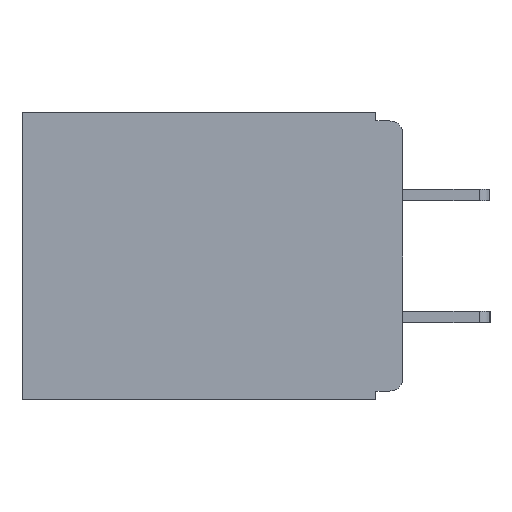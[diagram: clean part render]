
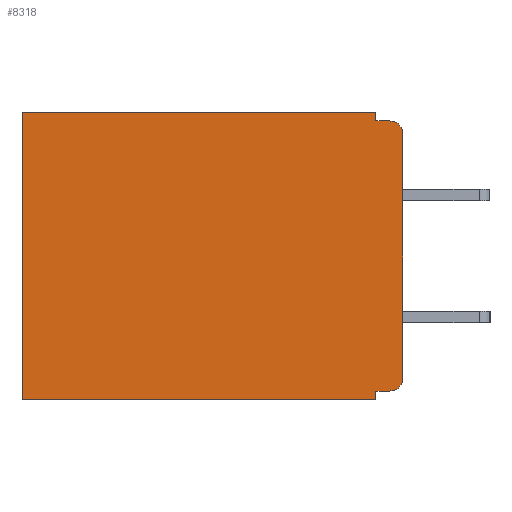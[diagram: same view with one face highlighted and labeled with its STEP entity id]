
A CAD part, left-side view. The second image highlights one B-rep face of the part: STEP entity #8318.
In plain terms, the highlighted planar face has unit normal (-1, 0, 0).
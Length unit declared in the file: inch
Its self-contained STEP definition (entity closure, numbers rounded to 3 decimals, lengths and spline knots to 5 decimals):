
#74 = CARTESIAN_POINT ( 'NONE',  ( 0.3, 0., -0.33 ) ) ;
#298 = ORIENTED_EDGE ( 'NONE', *, *, #14589, .F. ) ;
#323 = FACE_OUTER_BOUND ( 'NONE', #11181, .T. ) ;
#492 = CARTESIAN_POINT ( 'NONE',  ( 0.3, 0., 0. ) ) ;
#523 = DIRECTION ( 'NONE',  ( 0., 1., 0. ) ) ;
#769 = ORIENTED_EDGE ( 'NONE', *, *, #10823, .F. ) ;
#1187 = VERTEX_POINT ( 'NONE', #15953 ) ;
#1248 = ORIENTED_EDGE ( 'NONE', *, *, #4024, .T. ) ;
#2426 = ORIENTED_EDGE ( 'NONE', *, *, #8956, .T. ) ;
#2644 = VERTEX_POINT ( 'NONE', #4671 ) ;
#2681 = VERTEX_POINT ( 'NONE', #17995 ) ;
#2886 = ORIENTED_EDGE ( 'NONE', *, *, #8099, .F. ) ;
#3091 = VECTOR ( 'NONE', #6693, 39.37008 ) ;
#3391 = EDGE_CURVE ( 'NONE', #1187, #2681, #7046, .T. ) ;
#3652 = EDGE_CURVE ( 'NONE', #16773, #4041, #7027, .T. ) ;
#3713 = DIRECTION ( 'NONE',  ( 0., 0., -1. ) ) ;
#3838 = CARTESIAN_POINT ( 'NONE',  ( 0.3, 0.437, -0.33 ) ) ;
#4024 = EDGE_CURVE ( 'NONE', #2644, #4041, #8364, .T. ) ;
#4041 = VERTEX_POINT ( 'NONE', #16017 ) ;
#4089 = VECTOR ( 'NONE', #11317, 39.37008 ) ;
#4608 = VECTOR ( 'NONE', #8667, 39.37008 ) ;
#4671 = CARTESIAN_POINT ( 'NONE',  ( 0.3, 0.015, -0.32 ) ) ;
#5006 = VERTEX_POINT ( 'NONE', #17728 ) ;
#5085 = LINE ( 'NONE', #18104, #4608 ) ;
#5530 = EDGE_CURVE ( 'NONE', #2681, #14170, #16859, .T. ) ;
#5645 = DIRECTION ( 'NONE',  ( 0., 0., -1. ) ) ;
#6138 = DIRECTION ( 'NONE',  ( 0., 1., 0. ) ) ;
#6177 = EDGE_CURVE ( 'NONE', #14792, #16136, #17452, .T. ) ;
#6693 = DIRECTION ( 'NONE',  ( 0., 1., 0. ) ) ;
#7027 = LINE ( 'NONE', #74, #10357 ) ;
#7046 = LINE ( 'NONE', #492, #3091 ) ;
#7137 = CARTESIAN_POINT ( 'NONE',  ( 0.3, 0.031, -0.33 ) ) ;
#7290 = ORIENTED_EDGE ( 'NONE', *, *, #3391, .T. ) ;
#7534 = DIRECTION ( 'NONE',  ( 0., 0., -1. ) ) ;
#7620 = DIRECTION ( 'NONE',  ( 1., 0., 0. ) ) ;
#7642 = LINE ( 'NONE', #17520, #17646 ) ;
#7730 = CARTESIAN_POINT ( 'NONE',  ( 0.3, 0., -0.33 ) ) ;
#7813 = PLANE ( 'NONE',  #13607 ) ;
#8099 = EDGE_CURVE ( 'NONE', #1187, #12750, #11316, .T. ) ;
#8203 = LINE ( 'NONE', #14498, #15107 ) ;
#8318 = ADVANCED_FACE ( 'NONE', ( #323 ), #7813, .F. ) ;
#8364 = CIRCLE ( 'NONE', #11040, 0.015 ) ;
#8667 = DIRECTION ( 'NONE',  ( 0., -1., 0. ) ) ;
#8891 = CIRCLE ( 'NONE', #14738, 0.015 ) ;
#8956 = EDGE_CURVE ( 'NONE', #16773, #5006, #8891, .T. ) ;
#10357 = VECTOR ( 'NONE', #16633, 39.37008 ) ;
#10823 = EDGE_CURVE ( 'NONE', #2644, #14792, #8203, .T. ) ;
#11040 = AXIS2_PLACEMENT_3D ( 'NONE', #18044, #11717, #16079 ) ;
#11181 = EDGE_LOOP ( 'NONE', ( #16941, #2426, #17340, #2886, #7290, #18146, #298, #11937, #769, #1248 ) ) ;
#11316 = LINE ( 'NONE', #11357, #4089 ) ;
#11317 = DIRECTION ( 'NONE',  ( 0., 0., -1. ) ) ;
#11357 = CARTESIAN_POINT ( 'NONE',  ( 0.3, 0.031, 0. ) ) ;
#11717 = DIRECTION ( 'NONE',  ( -1., 0., 0. ) ) ;
#11937 = ORIENTED_EDGE ( 'NONE', *, *, #6177, .F. ) ;
#12648 = CARTESIAN_POINT ( 'NONE',  ( 0.3, 0.437, -0.33 ) ) ;
#12750 = VERTEX_POINT ( 'NONE', #14842 ) ;
#13193 = CARTESIAN_POINT ( 'NONE',  ( 0.3, 0.031, -0.33 ) ) ;
#13607 = AXIS2_PLACEMENT_3D ( 'NONE', #7730, #7620, #7534 ) ;
#13959 = VECTOR ( 'NONE', #5645, 39.37008 ) ;
#14170 = VERTEX_POINT ( 'NONE', #12648 ) ;
#14191 = VECTOR ( 'NONE', #3713, 39.37008 ) ;
#14498 = CARTESIAN_POINT ( 'NONE',  ( 0.3, 0., -0.32 ) ) ;
#14589 = EDGE_CURVE ( 'NONE', #16136, #14170, #7642, .T. ) ;
#14738 = AXIS2_PLACEMENT_3D ( 'NONE', #15737, #15732, #15708 ) ;
#14792 = VERTEX_POINT ( 'NONE', #15356 ) ;
#14842 = CARTESIAN_POINT ( 'NONE',  ( 0.3, 0.031, -0.01 ) ) ;
#15107 = VECTOR ( 'NONE', #6138, 39.37008 ) ;
#15149 = CARTESIAN_POINT ( 'NONE',  ( 0.3, 0., -0.025 ) ) ;
#15356 = CARTESIAN_POINT ( 'NONE',  ( 0.3, 0.031, -0.32 ) ) ;
#15388 = EDGE_CURVE ( 'NONE', #12750, #5006, #5085, .T. ) ;
#15708 = DIRECTION ( 'NONE',  ( 0., 0., -1. ) ) ;
#15732 = DIRECTION ( 'NONE',  ( -1., 0., 0. ) ) ;
#15737 = CARTESIAN_POINT ( 'NONE',  ( 0.3, 0.015, -0.025 ) ) ;
#15953 = CARTESIAN_POINT ( 'NONE',  ( 0.3, 0.031, 0. ) ) ;
#16017 = CARTESIAN_POINT ( 'NONE',  ( 0.3, 0., -0.305 ) ) ;
#16079 = DIRECTION ( 'NONE',  ( 0., 0., -1. ) ) ;
#16136 = VERTEX_POINT ( 'NONE', #13193 ) ;
#16633 = DIRECTION ( 'NONE',  ( 0., 0., -1. ) ) ;
#16773 = VERTEX_POINT ( 'NONE', #15149 ) ;
#16859 = LINE ( 'NONE', #3838, #14191 ) ;
#16941 = ORIENTED_EDGE ( 'NONE', *, *, #3652, .F. ) ;
#17340 = ORIENTED_EDGE ( 'NONE', *, *, #15388, .F. ) ;
#17452 = LINE ( 'NONE', #7137, #13959 ) ;
#17520 = CARTESIAN_POINT ( 'NONE',  ( 0.3, 0., -0.33 ) ) ;
#17646 = VECTOR ( 'NONE', #523, 39.37008 ) ;
#17728 = CARTESIAN_POINT ( 'NONE',  ( 0.3, 0.015, -0.01 ) ) ;
#17995 = CARTESIAN_POINT ( 'NONE',  ( 0.3, 0.437, 0. ) ) ;
#18044 = CARTESIAN_POINT ( 'NONE',  ( 0.3, 0.015, -0.305 ) ) ;
#18104 = CARTESIAN_POINT ( 'NONE',  ( 0.3, 0., -0.01 ) ) ;
#18146 = ORIENTED_EDGE ( 'NONE', *, *, #5530, .T. ) ;
